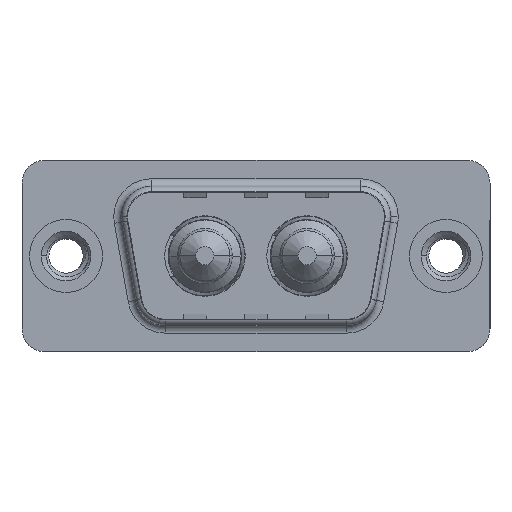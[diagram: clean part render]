
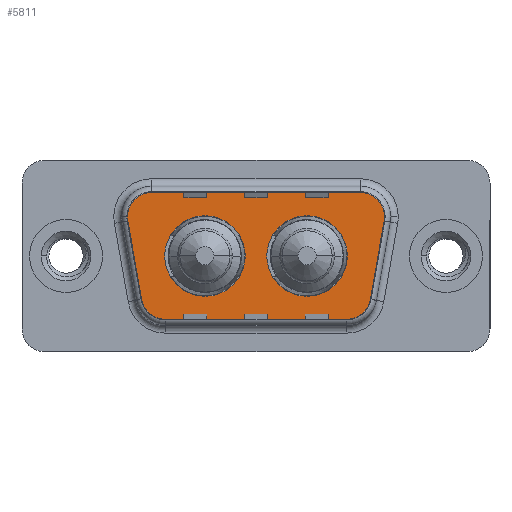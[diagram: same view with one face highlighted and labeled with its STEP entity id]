
A CAD part, top view. The second image highlights one B-rep face of the part: STEP entity #5811.
In plain terms, the highlighted planar face has unit normal (0, 0, 1).
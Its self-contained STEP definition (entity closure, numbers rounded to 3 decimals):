
#25 = DIRECTION ( 'NONE',  ( 1., 0., 0. ) ) ;
#33 = VECTOR ( 'NONE', #3814, 1000. ) ;
#512 = ORIENTED_EDGE ( 'NONE', *, *, #3045, .T. ) ;
#532 = CARTESIAN_POINT ( 'NONE',  ( 19.564, 4.9, 0. ) ) ;
#636 = AXIS2_PLACEMENT_3D ( 'NONE', #11690, #9954, #9941 ) ;
#695 = CARTESIAN_POINT ( 'NONE',  ( 21.534, 2.553, 0. ) ) ;
#752 = EDGE_CURVE ( 'NONE', #4084, #8038, #10450, .T. ) ;
#831 = CARTESIAN_POINT ( 'NONE',  ( 18.541, -2.9, 0. ) ) ;
#841 = DIRECTION ( 'NONE',  ( 0., 0., 1. ) ) ;
#1013 = EDGE_CURVE ( 'NONE', #4047, #8715, #2525, .T. ) ;
#1343 = DIRECTION ( 'NONE',  ( 0., 0., 1. ) ) ;
#1413 = CARTESIAN_POINT ( 'NONE',  ( 19.564, 2.9, 0. ) ) ;
#1623 = PLANE ( 'NONE',  #10560 ) ;
#1659 = VERTEX_POINT ( 'NONE', #2051 ) ;
#1662 = ORIENTED_EDGE ( 'NONE', *, *, #9069, .T. ) ;
#1831 = CARTESIAN_POINT ( 'NONE',  ( 5.436, 2.9, 0. ) ) ;
#2051 = CARTESIAN_POINT ( 'NONE',  ( 18.51, 0., 0. ) ) ;
#2059 = EDGE_CURVE ( 'NONE', #8715, #2285, #3573, .T. ) ;
#2090 = CARTESIAN_POINT ( 'NONE',  ( 20.511, -3.247, 0. ) ) ;
#2221 = CIRCLE ( 'NONE', #10278, 2. ) ;
#2285 = VERTEX_POINT ( 'NONE', #7149 ) ;
#2339 = DIRECTION ( 'NONE',  ( -1., 0., 0. ) ) ;
#2410 = DIRECTION ( 'NONE',  ( 0., 0., 1. ) ) ;
#2461 = VERTEX_POINT ( 'NONE', #4816 ) ;
#2512 = FACE_OUTER_BOUND ( 'NONE', #4754, .T. ) ;
#2514 = DIRECTION ( 'NONE',  ( 1., 0., 0. ) ) ;
#2525 = LINE ( 'NONE', #2968, #33 ) ;
#2721 = EDGE_CURVE ( 'NONE', #6999, #5747, #5489, .T. ) ;
#2913 = VERTEX_POINT ( 'NONE', #6174 ) ;
#2968 = CARTESIAN_POINT ( 'NONE',  ( 5.436, 4.9, 0. ) ) ;
#3040 = CARTESIAN_POINT ( 'NONE',  ( 9.14, 0., 0. ) ) ;
#3044 = EDGE_CURVE ( 'NONE', #1659, #2913, #11895, .T. ) ;
#3045 = EDGE_CURVE ( 'NONE', #8038, #3086, #2221, .T. ) ;
#3086 = VERTEX_POINT ( 'NONE', #10814 ) ;
#3289 = LINE ( 'NONE', #8425, #5524 ) ;
#3553 = DIRECTION ( 'NONE',  ( -1., 0., 0. ) ) ;
#3573 = CIRCLE ( 'NONE', #3944, 2. ) ;
#3628 = EDGE_LOOP ( 'NONE', ( #8693, #4292 ) ) ;
#3660 = EDGE_CURVE ( 'NONE', #2285, #8104, #3289, .T. ) ;
#3814 = DIRECTION ( 'NONE',  ( -1., 0., 0. ) ) ;
#3831 = AXIS2_PLACEMENT_3D ( 'NONE', #11270, #5694, #25 ) ;
#3938 = CARTESIAN_POINT ( 'NONE',  ( 6.49, 0., 0. ) ) ;
#3944 = AXIS2_PLACEMENT_3D ( 'NONE', #1831, #841, #5522 ) ;
#3952 = ORIENTED_EDGE ( 'NONE', *, *, #9808, .T. ) ;
#3959 = DIRECTION ( 'NONE',  ( 0., 0., 1. ) ) ;
#4047 = VERTEX_POINT ( 'NONE', #532 ) ;
#4084 = VERTEX_POINT ( 'NONE', #2090 ) ;
#4099 = ORIENTED_EDGE ( 'NONE', *, *, #5482, .T. ) ;
#4209 = DIRECTION ( 'NONE',  ( 0.174, 0.985, 0. ) ) ;
#4289 = DIRECTION ( 'NONE',  ( 0., 0., 1. ) ) ;
#4292 = ORIENTED_EDGE ( 'NONE', *, *, #2721, .F. ) ;
#4739 = CARTESIAN_POINT ( 'NONE',  ( 18.541, -4.9, 0. ) ) ;
#4750 = EDGE_CURVE ( 'NONE', #5747, #6999, #10007, .T. ) ;
#4754 = EDGE_LOOP ( 'NONE', ( #11933, #11812, #512, #3952, #5267, #5931, #6045, #1662, #4099 ) ) ;
#4816 = CARTESIAN_POINT ( 'NONE',  ( 6.459, -4.9, 0. ) ) ;
#4822 = CARTESIAN_POINT ( 'NONE',  ( 11.79, 0., 0. ) ) ;
#4846 = DIRECTION ( 'NONE',  ( 1., 0., 0. ) ) ;
#4907 = VECTOR ( 'NONE', #4209, 1000. ) ;
#5038 = FACE_BOUND ( 'NONE', #10006, .T. ) ;
#5044 = DIRECTION ( 'NONE',  ( 0., 0., 1. ) ) ;
#5202 = DIRECTION ( 'NONE',  ( 1., 0., 0. ) ) ;
#5267 = ORIENTED_EDGE ( 'NONE', *, *, #1013, .T. ) ;
#5482 = EDGE_CURVE ( 'NONE', #2461, #11517, #8533, .T. ) ;
#5489 = CIRCLE ( 'NONE', #7241, 2.65 ) ;
#5522 = DIRECTION ( 'NONE',  ( 1., 0., 0. ) ) ;
#5524 = VECTOR ( 'NONE', #9532, 1000. ) ;
#5694 = DIRECTION ( 'NONE',  ( 0., 0., 1. ) ) ;
#5747 = VERTEX_POINT ( 'NONE', #4822 ) ;
#5811 = ADVANCED_FACE ( 'NONE', ( #5038, #7512, #2512 ), #1623, .T. ) ;
#5931 = ORIENTED_EDGE ( 'NONE', *, *, #2059, .T. ) ;
#6045 = ORIENTED_EDGE ( 'NONE', *, *, #3660, .T. ) ;
#6174 = CARTESIAN_POINT ( 'NONE',  ( 13.21, 0., 0. ) ) ;
#6282 = EDGE_CURVE ( 'NONE', #2913, #1659, #10564, .T. ) ;
#6390 = ORIENTED_EDGE ( 'NONE', *, *, #6282, .F. ) ;
#6633 = CARTESIAN_POINT ( 'NONE',  ( 19.564, 2.9, 0. ) ) ;
#6865 = ORIENTED_EDGE ( 'NONE', *, *, #3044, .F. ) ;
#6968 = CARTESIAN_POINT ( 'NONE',  ( 15.86, 0., 0. ) ) ;
#6999 = VERTEX_POINT ( 'NONE', #3938 ) ;
#7149 = CARTESIAN_POINT ( 'NONE',  ( 3.466, 2.553, 0. ) ) ;
#7180 = DIRECTION ( 'NONE',  ( 0., 0., 1. ) ) ;
#7241 = AXIS2_PLACEMENT_3D ( 'NONE', #3040, #4289, #5202 ) ;
#7285 = CIRCLE ( 'NONE', #11877, 2. ) ;
#7512 = FACE_BOUND ( 'NONE', #3628, .T. ) ;
#7558 = CIRCLE ( 'NONE', #7639, 2. ) ;
#7639 = AXIS2_PLACEMENT_3D ( 'NONE', #9549, #3959, #10493 ) ;
#7940 = DIRECTION ( 'NONE',  ( 0., 0., 1. ) ) ;
#8038 = VERTEX_POINT ( 'NONE', #9752 ) ;
#8104 = VERTEX_POINT ( 'NONE', #10894 ) ;
#8425 = CARTESIAN_POINT ( 'NONE',  ( 3.466, 2.553, 0. ) ) ;
#8533 = LINE ( 'NONE', #9849, #10738 ) ;
#8656 = AXIS2_PLACEMENT_3D ( 'NONE', #1413, #7940, #2339 ) ;
#8693 = ORIENTED_EDGE ( 'NONE', *, *, #4750, .F. ) ;
#8715 = VERTEX_POINT ( 'NONE', #11996 ) ;
#9042 = AXIS2_PLACEMENT_3D ( 'NONE', #6968, #7180, #4846 ) ;
#9069 = EDGE_CURVE ( 'NONE', #8104, #2461, #7285, .T. ) ;
#9532 = DIRECTION ( 'NONE',  ( 0.174, -0.985, 0. ) ) ;
#9549 = CARTESIAN_POINT ( 'NONE',  ( 18.541, -2.9, 0. ) ) ;
#9616 = EDGE_CURVE ( 'NONE', #11517, #4084, #7558, .T. ) ;
#9752 = CARTESIAN_POINT ( 'NONE',  ( 21.534, 2.553, 0. ) ) ;
#9808 = EDGE_CURVE ( 'NONE', #3086, #4047, #10774, .T. ) ;
#9849 = CARTESIAN_POINT ( 'NONE',  ( 6.459, -4.9, 0. ) ) ;
#9941 = DIRECTION ( 'NONE',  ( 1., 0., 0. ) ) ;
#9954 = DIRECTION ( 'NONE',  ( 0., 0., 1. ) ) ;
#9963 = DIRECTION ( 'NONE',  ( 1., 0., 0. ) ) ;
#10006 = EDGE_LOOP ( 'NONE', ( #6865, #6390 ) ) ;
#10007 = CIRCLE ( 'NONE', #636, 2.65 ) ;
#10278 = AXIS2_PLACEMENT_3D ( 'NONE', #6633, #2410, #3553 ) ;
#10450 = LINE ( 'NONE', #695, #4907 ) ;
#10493 = DIRECTION ( 'NONE',  ( 1., 0., 0. ) ) ;
#10560 = AXIS2_PLACEMENT_3D ( 'NONE', #831, #1343, #2514 ) ;
#10564 = CIRCLE ( 'NONE', #3831, 2.65 ) ;
#10633 = CARTESIAN_POINT ( 'NONE',  ( 6.459, -2.9, 0. ) ) ;
#10738 = VECTOR ( 'NONE', #9963, 1000. ) ;
#10774 = CIRCLE ( 'NONE', #8656, 2. ) ;
#10814 = CARTESIAN_POINT ( 'NONE',  ( 21.564, 2.9, 0. ) ) ;
#10894 = CARTESIAN_POINT ( 'NONE',  ( 4.489, -3.247, 0. ) ) ;
#11270 = CARTESIAN_POINT ( 'NONE',  ( 15.86, 0., 0. ) ) ;
#11517 = VERTEX_POINT ( 'NONE', #4739 ) ;
#11578 = DIRECTION ( 'NONE',  ( -1., 0., 0. ) ) ;
#11690 = CARTESIAN_POINT ( 'NONE',  ( 9.14, 0., 0. ) ) ;
#11812 = ORIENTED_EDGE ( 'NONE', *, *, #752, .T. ) ;
#11877 = AXIS2_PLACEMENT_3D ( 'NONE', #10633, #5044, #11578 ) ;
#11895 = CIRCLE ( 'NONE', #9042, 2.65 ) ;
#11933 = ORIENTED_EDGE ( 'NONE', *, *, #9616, .T. ) ;
#11996 = CARTESIAN_POINT ( 'NONE',  ( 5.436, 4.9, 0. ) ) ;
